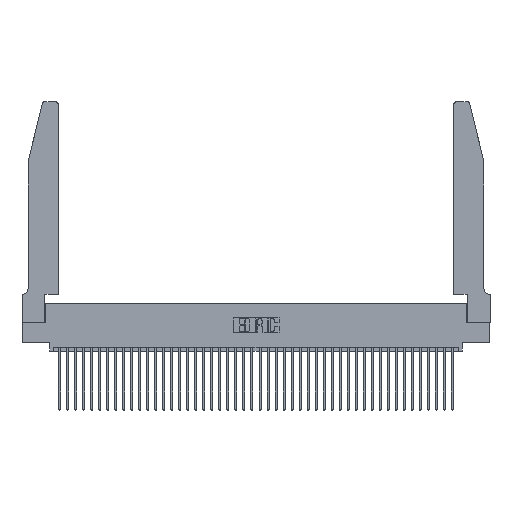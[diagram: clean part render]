
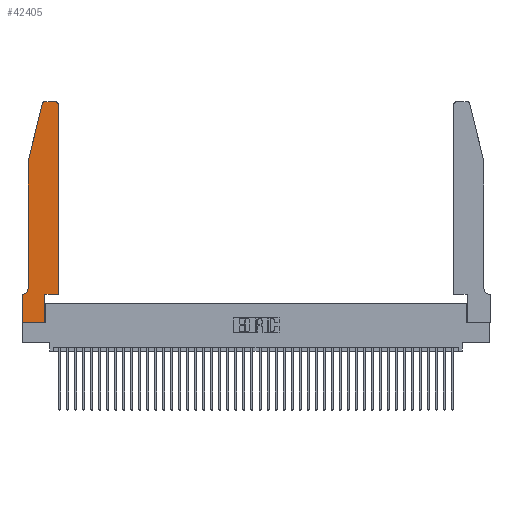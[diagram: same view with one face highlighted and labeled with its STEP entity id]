
A CAD part, top view. The second image highlights one B-rep face of the part: STEP entity #42405.
In plain terms, the highlighted planar face has unit normal (0, 0, 1).
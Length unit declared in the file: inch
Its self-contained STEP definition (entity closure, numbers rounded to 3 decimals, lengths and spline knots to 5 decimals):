
#927 = ORIENTED_EDGE ( 'NONE', *, *, #3277, .T. ) ;
#1143 = LINE ( 'NONE', #6524, #26819 ) ;
#1189 = ORIENTED_EDGE ( 'NONE', *, *, #31366, .T. ) ;
#1243 = VERTEX_POINT ( 'NONE', #21841 ) ;
#1635 = EDGE_CURVE ( 'NONE', #7058, #33473, #41011, .T. ) ;
#2152 = LINE ( 'NONE', #23236, #36535 ) ;
#2474 = CARTESIAN_POINT ( 'NONE',  ( 0.4505, 0.35, 0.37 ) ) ;
#3277 = EDGE_CURVE ( 'NONE', #10482, #7058, #12936, .T. ) ;
#3514 = VERTEX_POINT ( 'NONE', #25742 ) ;
#3716 = LINE ( 'NONE', #11075, #11634 ) ;
#3816 = CARTESIAN_POINT ( 'NONE',  ( 0., 0.35, 0.37 ) ) ;
#4932 = ORIENTED_EDGE ( 'NONE', *, *, #6946, .T. ) ;
#5410 = VECTOR ( 'NONE', #12209, 39.37008 ) ;
#5726 = LINE ( 'NONE', #2474, #12565 ) ;
#6089 = AXIS2_PLACEMENT_3D ( 'NONE', #32831, #12944, #36112 ) ;
#6184 = CARTESIAN_POINT ( 'NONE',  ( 0.4205, 2.75, 0.37 ) ) ;
#6510 = ORIENTED_EDGE ( 'NONE', *, *, #38979, .T. ) ;
#6524 = CARTESIAN_POINT ( 'NONE',  ( 0.0755, 0.35, 0.37 ) ) ;
#6910 = ORIENTED_EDGE ( 'NONE', *, *, #38926, .T. ) ;
#6946 = EDGE_CURVE ( 'NONE', #33473, #24960, #3716, .T. ) ;
#7058 = VERTEX_POINT ( 'NONE', #8404 ) ;
#7365 = DIRECTION ( 'NONE',  ( 0., 0., 1. ) ) ;
#7974 = VECTOR ( 'NONE', #13947, 39.37008 ) ;
#8404 = CARTESIAN_POINT ( 'NONE',  ( 0., 0., 0.37 ) ) ;
#8832 = ORIENTED_EDGE ( 'NONE', *, *, #25168, .T. ) ;
#8956 = VERTEX_POINT ( 'NONE', #18375 ) ;
#9193 = ORIENTED_EDGE ( 'NONE', *, *, #1635, .T. ) ;
#10144 = VERTEX_POINT ( 'NONE', #34338 ) ;
#10180 = CARTESIAN_POINT ( 'NONE',  ( 0., 0., 0.37 ) ) ;
#10482 = VERTEX_POINT ( 'NONE', #22743 ) ;
#11075 = CARTESIAN_POINT ( 'NONE',  ( 0.2865, 0.35, 0.37 ) ) ;
#11193 = CARTESIAN_POINT ( 'NONE',  ( 0., 0., 0.37 ) ) ;
#11196 = VERTEX_POINT ( 'NONE', #6184 ) ;
#11305 = VERTEX_POINT ( 'NONE', #33229 ) ;
#11634 = VECTOR ( 'NONE', #21102, 39.37008 ) ;
#12209 = DIRECTION ( 'NONE',  ( -1., 0., 0. ) ) ;
#12565 = VECTOR ( 'NONE', #29229, 39.37008 ) ;
#12848 = EDGE_CURVE ( 'NONE', #11196, #23060, #30965, .T. ) ;
#12936 = LINE ( 'NONE', #11193, #39331 ) ;
#12944 = DIRECTION ( 'NONE',  ( 0., 0., -1. ) ) ;
#12999 = EDGE_CURVE ( 'NONE', #20909, #11196, #27844, .T. ) ;
#13090 = DIRECTION ( 'NONE',  ( 0., 0., 1. ) ) ;
#13947 = DIRECTION ( 'NONE',  ( 0., -1., 0. ) ) ;
#14790 = CARTESIAN_POINT ( 'NONE',  ( 0.4505, 2.72, 0.37 ) ) ;
#15695 = VECTOR ( 'NONE', #39990, 39.37008 ) ;
#15791 = EDGE_LOOP ( 'NONE', ( #40033, #26311, #8832, #23888, #6510, #1189, #927, #9193, #4932, #30202, #6910, #42928 ) ) ;
#16411 = FACE_OUTER_BOUND ( 'NONE', #15791, .T. ) ;
#17167 = CARTESIAN_POINT ( 'NONE',  ( 0.284, 2.72, 0.37 ) ) ;
#17282 = LINE ( 'NONE', #25966, #26106 ) ;
#17913 = DIRECTION ( 'NONE',  ( 0., -1., 0. ) ) ;
#18375 = CARTESIAN_POINT ( 'NONE',  ( 0.0755, 2., 0.37 ) ) ;
#20461 = DIRECTION ( 'NONE',  ( 1., 0., 0. ) ) ;
#20909 = VERTEX_POINT ( 'NONE', #14790 ) ;
#21102 = DIRECTION ( 'NONE',  ( 0., 1., 0. ) ) ;
#21841 = CARTESIAN_POINT ( 'NONE',  ( 0.0755, 0.42, 0.37 ) ) ;
#21893 = CIRCLE ( 'NONE', #28442, 0.03 ) ;
#22743 = CARTESIAN_POINT ( 'NONE',  ( 0., 0.35, 0.37 ) ) ;
#22865 = EDGE_CURVE ( 'NONE', #8956, #1243, #27791, .T. ) ;
#23060 = VERTEX_POINT ( 'NONE', #28441 ) ;
#23236 = CARTESIAN_POINT ( 'NONE',  ( 0.4505, 0.35, 0.37 ) ) ;
#23888 = ORIENTED_EDGE ( 'NONE', *, *, #22865, .T. ) ;
#24378 = AXIS2_PLACEMENT_3D ( 'NONE', #32967, #13090, #36246 ) ;
#24960 = VERTEX_POINT ( 'NONE', #37927 ) ;
#25168 = EDGE_CURVE ( 'NONE', #3514, #8956, #17282, .T. ) ;
#25742 = CARTESIAN_POINT ( 'NONE',  ( 0.25487, 2.72718, 0.37 ) ) ;
#25966 = CARTESIAN_POINT ( 'NONE',  ( 0.0755, 2., 0.37 ) ) ;
#26106 = VECTOR ( 'NONE', #29310, 39.37008 ) ;
#26311 = ORIENTED_EDGE ( 'NONE', *, *, #39161, .T. ) ;
#26819 = VECTOR ( 'NONE', #33565, 39.37008 ) ;
#27349 = PLANE ( 'NONE',  #29073 ) ;
#27791 = LINE ( 'NONE', #30472, #7974 ) ;
#27844 = CIRCLE ( 'NONE', #24378, 0.03 ) ;
#28441 = CARTESIAN_POINT ( 'NONE',  ( 0.284, 2.75, 0.37 ) ) ;
#28442 = AXIS2_PLACEMENT_3D ( 'NONE', #17167, #40237, #20461 ) ;
#29073 = AXIS2_PLACEMENT_3D ( 'NONE', #3816, #7365, #30674 ) ;
#29206 = CIRCLE ( 'NONE', #6089, 0.07 ) ;
#29229 = DIRECTION ( 'NONE',  ( 0., 1., 0. ) ) ;
#29310 = DIRECTION ( 'NONE',  ( -0.239, -0.971, 0. ) ) ;
#30061 = DIRECTION ( 'NONE',  ( 1., 0., 0. ) ) ;
#30202 = ORIENTED_EDGE ( 'NONE', *, *, #42965, .T. ) ;
#30472 = CARTESIAN_POINT ( 'NONE',  ( 0.0755, 2., 0.37 ) ) ;
#30674 = DIRECTION ( 'NONE',  ( 1., 0., 0. ) ) ;
#30965 = LINE ( 'NONE', #32121, #5410 ) ;
#31366 = EDGE_CURVE ( 'NONE', #11305, #10482, #1143, .T. ) ;
#31411 = CARTESIAN_POINT ( 'NONE',  ( 0.2865, 0., 0.37 ) ) ;
#32121 = CARTESIAN_POINT ( 'NONE',  ( 0.2605, 2.75, 0.37 ) ) ;
#32831 = CARTESIAN_POINT ( 'NONE',  ( 0.0055, 0.42, 0.37 ) ) ;
#32967 = CARTESIAN_POINT ( 'NONE',  ( 0.4205, 2.72, 0.37 ) ) ;
#33229 = CARTESIAN_POINT ( 'NONE',  ( 0.0055, 0.35, 0.37 ) ) ;
#33473 = VERTEX_POINT ( 'NONE', #31411 ) ;
#33565 = DIRECTION ( 'NONE',  ( -1., 0., 0. ) ) ;
#34338 = CARTESIAN_POINT ( 'NONE',  ( 0.4505, 0.35, 0.37 ) ) ;
#36112 = DIRECTION ( 'NONE',  ( -1., 0., 0. ) ) ;
#36246 = DIRECTION ( 'NONE',  ( 1., 0., 0. ) ) ;
#36535 = VECTOR ( 'NONE', #30061, 39.37008 ) ;
#37927 = CARTESIAN_POINT ( 'NONE',  ( 0.2865, 0.35, 0.37 ) ) ;
#38926 = EDGE_CURVE ( 'NONE', #10144, #20909, #5726, .T. ) ;
#38979 = EDGE_CURVE ( 'NONE', #1243, #11305, #29206, .T. ) ;
#39161 = EDGE_CURVE ( 'NONE', #23060, #3514, #21893, .T. ) ;
#39331 = VECTOR ( 'NONE', #17913, 39.37008 ) ;
#39990 = DIRECTION ( 'NONE',  ( 1., 0., 0. ) ) ;
#40033 = ORIENTED_EDGE ( 'NONE', *, *, #12848, .T. ) ;
#40237 = DIRECTION ( 'NONE',  ( 0., 0., 1. ) ) ;
#41011 = LINE ( 'NONE', #10180, #15695 ) ;
#42405 = ADVANCED_FACE ( 'NONE', ( #16411 ), #27349, .T. ) ;
#42928 = ORIENTED_EDGE ( 'NONE', *, *, #12999, .T. ) ;
#42965 = EDGE_CURVE ( 'NONE', #24960, #10144, #2152, .T. ) ;
